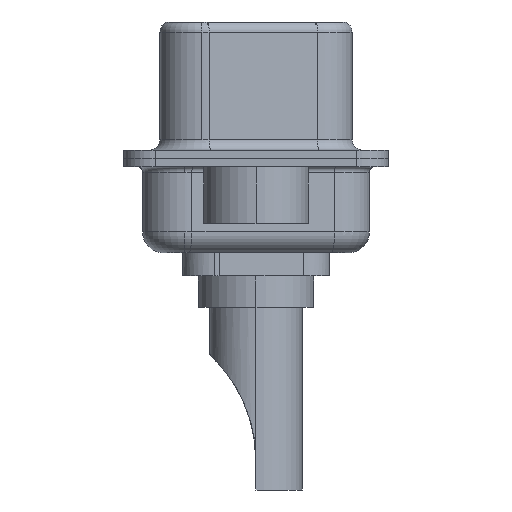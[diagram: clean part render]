
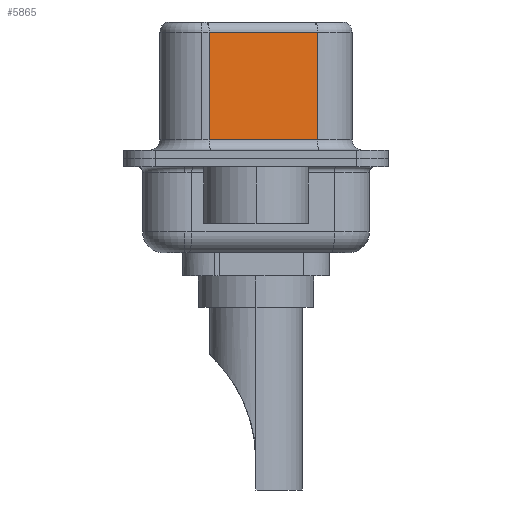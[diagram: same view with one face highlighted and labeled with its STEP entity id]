
A CAD part, left-side view. The second image highlights one B-rep face of the part: STEP entity #5865.
In plain terms, the highlighted planar face has unit normal (-0.985, -0.174, 0).
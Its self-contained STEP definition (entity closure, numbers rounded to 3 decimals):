
#790 = DIRECTION ( 'NONE',  ( 0., 0., -1. ) ) ;
#1319 = ORIENTED_EDGE ( 'NONE', *, *, #16015, .T. ) ;
#1643 = LINE ( 'NONE', #19161, #17294 ) ;
#1954 = EDGE_LOOP ( 'NONE', ( #21346, #9002, #1319, #4542 ) ) ;
#3177 = PLANE ( 'NONE',  #5053 ) ;
#3849 = VERTEX_POINT ( 'NONE', #18024 ) ;
#4423 = CARTESIAN_POINT ( 'NONE',  ( 4.58, -2.927, 0.9 ) ) ;
#4542 = ORIENTED_EDGE ( 'NONE', *, *, #10840, .T. ) ;
#5053 = AXIS2_PLACEMENT_3D ( 'NONE', #14756, #23675, #10164 ) ;
#5776 = LINE ( 'NONE', #23487, #17253 ) ;
#5865 = ADVANCED_FACE ( 'NONE', ( #10587 ), #3177, .F. ) ;
#6603 = VECTOR ( 'NONE', #18641, 1000. ) ;
#7352 = CARTESIAN_POINT ( 'NONE',  ( 3.67, 2.233, 0.9 ) ) ;
#9002 = ORIENTED_EDGE ( 'NONE', *, *, #11913, .T. ) ;
#10164 = DIRECTION ( 'NONE',  ( -0.174, 0.985, 0. ) ) ;
#10587 = FACE_OUTER_BOUND ( 'NONE', #1954, .T. ) ;
#10774 = CARTESIAN_POINT ( 'NONE',  ( 3.67, 2.233, 6.02 ) ) ;
#10840 = EDGE_CURVE ( 'NONE', #18422, #3849, #17427, .T. ) ;
#11374 = DIRECTION ( 'NONE',  ( 0., 0., -1. ) ) ;
#11913 = EDGE_CURVE ( 'NONE', #16846, #18758, #14526, .T. ) ;
#13881 = VECTOR ( 'NONE', #17460, 1000. ) ;
#14526 = LINE ( 'NONE', #15394, #13881 ) ;
#14756 = CARTESIAN_POINT ( 'NONE',  ( 4.58, -2.927, 6.52 ) ) ;
#14917 = EDGE_CURVE ( 'NONE', #16846, #3849, #1643, .T. ) ;
#15394 = CARTESIAN_POINT ( 'NONE',  ( 4.58, -2.927, 6.02 ) ) ;
#16015 = EDGE_CURVE ( 'NONE', #18758, #18422, #5776, .T. ) ;
#16846 = VERTEX_POINT ( 'NONE', #19936 ) ;
#17253 = VECTOR ( 'NONE', #11374, 1000. ) ;
#17294 = VECTOR ( 'NONE', #790, 1000. ) ;
#17427 = LINE ( 'NONE', #4423, #6603 ) ;
#17460 = DIRECTION ( 'NONE',  ( -0.174, 0.985, 0. ) ) ;
#18024 = CARTESIAN_POINT ( 'NONE',  ( 4.58, -2.927, 0.9 ) ) ;
#18422 = VERTEX_POINT ( 'NONE', #7352 ) ;
#18641 = DIRECTION ( 'NONE',  ( 0.174, -0.985, 0. ) ) ;
#18758 = VERTEX_POINT ( 'NONE', #10774 ) ;
#19161 = CARTESIAN_POINT ( 'NONE',  ( 4.58, -2.927, 6.52 ) ) ;
#19936 = CARTESIAN_POINT ( 'NONE',  ( 4.58, -2.927, 6.02 ) ) ;
#21346 = ORIENTED_EDGE ( 'NONE', *, *, #14917, .F. ) ;
#23487 = CARTESIAN_POINT ( 'NONE',  ( 3.67, 2.233, 6.52 ) ) ;
#23675 = DIRECTION ( 'NONE',  ( 0.985, 0.174, 0. ) ) ;
